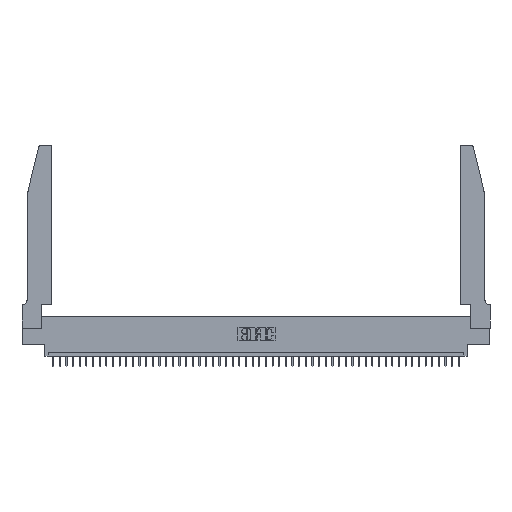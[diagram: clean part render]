
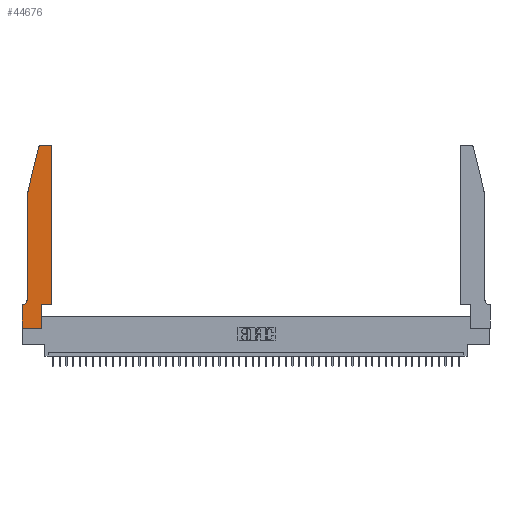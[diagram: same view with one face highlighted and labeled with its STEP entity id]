
A CAD part, top view. The second image highlights one B-rep face of the part: STEP entity #44676.
In plain terms, the highlighted planar face has unit normal (0, 0, 1).
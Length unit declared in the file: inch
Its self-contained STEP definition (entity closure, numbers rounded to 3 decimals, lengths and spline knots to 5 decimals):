
#23 = LINE ( 'NONE', #32280, #37857 ) ;
#699 = EDGE_CURVE ( 'NONE', #25619, #17878, #11691, .T. ) ;
#874 = ORIENTED_EDGE ( 'NONE', *, *, #14093, .T. ) ;
#895 = CARTESIAN_POINT ( 'NONE',  ( 0.25487, 2.72718, 0.37 ) ) ;
#1100 = CARTESIAN_POINT ( 'NONE',  ( 0.2865, 0.35, 0.37 ) ) ;
#2449 = VERTEX_POINT ( 'NONE', #40397 ) ;
#2462 = CARTESIAN_POINT ( 'NONE',  ( 0.4505, 0.35, 0.37 ) ) ;
#2941 = ORIENTED_EDGE ( 'NONE', *, *, #3847, .T. ) ;
#3013 = DIRECTION ( 'NONE',  ( 0., 1., 0. ) ) ;
#3695 = ORIENTED_EDGE ( 'NONE', *, *, #42398, .T. ) ;
#3847 = EDGE_CURVE ( 'NONE', #35915, #27266, #47450, .T. ) ;
#4477 = AXIS2_PLACEMENT_3D ( 'NONE', #24821, #9919, #25151 ) ;
#4875 = CARTESIAN_POINT ( 'NONE',  ( 0.0755, 0.42, 0.37 ) ) ;
#5432 = EDGE_LOOP ( 'NONE', ( #874, #41596, #39174, #23337, #21765, #13843, #41439, #3695, #14751, #2941, #32762, #30249 ) ) ;
#6868 = DIRECTION ( 'NONE',  ( -1., 0., 0. ) ) ;
#6948 = DIRECTION ( 'NONE',  ( 0., 1., 0. ) ) ;
#7345 = CARTESIAN_POINT ( 'NONE',  ( 0.4505, 0.35, 0.37 ) ) ;
#7988 = DIRECTION ( 'NONE',  ( 0., -1., 0. ) ) ;
#8310 = CARTESIAN_POINT ( 'NONE',  ( 0.284, 2.75, 0.37 ) ) ;
#8415 = VECTOR ( 'NONE', #6868, 39.37008 ) ;
#8465 = DIRECTION ( 'NONE',  ( 0., 0., 1. ) ) ;
#8596 = CIRCLE ( 'NONE', #4477, 0.03 ) ;
#8903 = EDGE_CURVE ( 'NONE', #35233, #26789, #16648, .T. ) ;
#9687 = VERTEX_POINT ( 'NONE', #895 ) ;
#9919 = DIRECTION ( 'NONE',  ( 0., 0., 1. ) ) ;
#10897 = LINE ( 'NONE', #25652, #37524 ) ;
#11164 = DIRECTION ( 'NONE',  ( -0.239, -0.971, 0. ) ) ;
#11323 = CARTESIAN_POINT ( 'NONE',  ( 0.0755, 2., 0.37 ) ) ;
#11691 = LINE ( 'NONE', #21975, #24125 ) ;
#12557 = DIRECTION ( 'NONE',  ( -1., 0., 0. ) ) ;
#13031 = VECTOR ( 'NONE', #11164, 39.37008 ) ;
#13135 = DIRECTION ( 'NONE',  ( 0., 0., -1. ) ) ;
#13655 = VERTEX_POINT ( 'NONE', #8310 ) ;
#13843 = ORIENTED_EDGE ( 'NONE', *, *, #21117, .T. ) ;
#14093 = EDGE_CURVE ( 'NONE', #30449, #13655, #48654, .T. ) ;
#14190 = VECTOR ( 'NONE', #26966, 39.37008 ) ;
#14314 = DIRECTION ( 'NONE',  ( 0., 0., 1. ) ) ;
#14751 = ORIENTED_EDGE ( 'NONE', *, *, #24296, .T. ) ;
#14823 = DIRECTION ( 'NONE',  ( -1., 0., 0. ) ) ;
#15380 = CARTESIAN_POINT ( 'NONE',  ( 0.4505, 0.35, 0.37 ) ) ;
#15409 = VECTOR ( 'NONE', #3013, 39.37008 ) ;
#16256 = EDGE_CURVE ( 'NONE', #13655, #9687, #17900, .T. ) ;
#16648 = LINE ( 'NONE', #24635, #34934 ) ;
#17878 = VERTEX_POINT ( 'NONE', #4875 ) ;
#17900 = CIRCLE ( 'NONE', #21139, 0.03 ) ;
#17932 = VECTOR ( 'NONE', #18370, 39.37008 ) ;
#18126 = CARTESIAN_POINT ( 'NONE',  ( 0.2605, 2.75, 0.37 ) ) ;
#18370 = DIRECTION ( 'NONE',  ( 1., 0., 0. ) ) ;
#21102 = VERTEX_POINT ( 'NONE', #45766 ) ;
#21117 = EDGE_CURVE ( 'NONE', #35911, #35233, #23, .T. ) ;
#21139 = AXIS2_PLACEMENT_3D ( 'NONE', #23509, #8465, #34865 ) ;
#21765 = ORIENTED_EDGE ( 'NONE', *, *, #27691, .T. ) ;
#21975 = CARTESIAN_POINT ( 'NONE',  ( 0.0755, 2., 0.37 ) ) ;
#22614 = CIRCLE ( 'NONE', #40969, 0.07 ) ;
#23056 = LINE ( 'NONE', #11323, #13031 ) ;
#23190 = CARTESIAN_POINT ( 'NONE',  ( 0., 0., 0.37 ) ) ;
#23337 = ORIENTED_EDGE ( 'NONE', *, *, #699, .T. ) ;
#23509 = CARTESIAN_POINT ( 'NONE',  ( 0.284, 2.72, 0.37 ) ) ;
#24125 = VECTOR ( 'NONE', #7988, 39.37008 ) ;
#24296 = EDGE_CURVE ( 'NONE', #2449, #35915, #10897, .T. ) ;
#24635 = CARTESIAN_POINT ( 'NONE',  ( 0., 0., 0.37 ) ) ;
#24821 = CARTESIAN_POINT ( 'NONE',  ( 0.4205, 2.72, 0.37 ) ) ;
#25151 = DIRECTION ( 'NONE',  ( 1., 0., 0. ) ) ;
#25487 = LINE ( 'NONE', #7345, #15409 ) ;
#25619 = VERTEX_POINT ( 'NONE', #39149 ) ;
#25652 = CARTESIAN_POINT ( 'NONE',  ( 0.2865, 0.35, 0.37 ) ) ;
#26789 = VERTEX_POINT ( 'NONE', #44577 ) ;
#26958 = AXIS2_PLACEMENT_3D ( 'NONE', #40767, #14314, #44571 ) ;
#26966 = DIRECTION ( 'NONE',  ( 1., 0., 0. ) ) ;
#27266 = VERTEX_POINT ( 'NONE', #2462 ) ;
#27691 = EDGE_CURVE ( 'NONE', #17878, #35911, #22614, .T. ) ;
#29568 = LINE ( 'NONE', #23190, #14190 ) ;
#30249 = ORIENTED_EDGE ( 'NONE', *, *, #39207, .T. ) ;
#30449 = VERTEX_POINT ( 'NONE', #38859 ) ;
#30717 = FACE_OUTER_BOUND ( 'NONE', #5432, .T. ) ;
#31787 = CARTESIAN_POINT ( 'NONE',  ( 0.0055, 0.42, 0.37 ) ) ;
#32280 = CARTESIAN_POINT ( 'NONE',  ( 0.0755, 0.35, 0.37 ) ) ;
#32762 = ORIENTED_EDGE ( 'NONE', *, *, #42264, .T. ) ;
#34865 = DIRECTION ( 'NONE',  ( 1., 0., 0. ) ) ;
#34934 = VECTOR ( 'NONE', #41010, 39.37008 ) ;
#35233 = VERTEX_POINT ( 'NONE', #47978 ) ;
#35841 = CARTESIAN_POINT ( 'NONE',  ( 0.0055, 0.35, 0.37 ) ) ;
#35911 = VERTEX_POINT ( 'NONE', #35841 ) ;
#35915 = VERTEX_POINT ( 'NONE', #1100 ) ;
#37524 = VECTOR ( 'NONE', #6948, 39.37008 ) ;
#37857 = VECTOR ( 'NONE', #12557, 39.37008 ) ;
#38859 = CARTESIAN_POINT ( 'NONE',  ( 0.4205, 2.75, 0.37 ) ) ;
#39149 = CARTESIAN_POINT ( 'NONE',  ( 0.0755, 2., 0.37 ) ) ;
#39174 = ORIENTED_EDGE ( 'NONE', *, *, #44703, .T. ) ;
#39207 = EDGE_CURVE ( 'NONE', #21102, #30449, #8596, .T. ) ;
#40397 = CARTESIAN_POINT ( 'NONE',  ( 0.2865, 0., 0.37 ) ) ;
#40767 = CARTESIAN_POINT ( 'NONE',  ( 0., 0.35, 0.37 ) ) ;
#40944 = PLANE ( 'NONE',  #26958 ) ;
#40969 = AXIS2_PLACEMENT_3D ( 'NONE', #31787, #13135, #14823 ) ;
#41010 = DIRECTION ( 'NONE',  ( 0., -1., 0. ) ) ;
#41439 = ORIENTED_EDGE ( 'NONE', *, *, #8903, .T. ) ;
#41596 = ORIENTED_EDGE ( 'NONE', *, *, #16256, .T. ) ;
#42264 = EDGE_CURVE ( 'NONE', #27266, #21102, #25487, .T. ) ;
#42398 = EDGE_CURVE ( 'NONE', #26789, #2449, #29568, .T. ) ;
#44571 = DIRECTION ( 'NONE',  ( 1., 0., 0. ) ) ;
#44577 = CARTESIAN_POINT ( 'NONE',  ( 0., 0., 0.37 ) ) ;
#44676 = ADVANCED_FACE ( 'NONE', ( #30717 ), #40944, .T. ) ;
#44703 = EDGE_CURVE ( 'NONE', #9687, #25619, #23056, .T. ) ;
#45766 = CARTESIAN_POINT ( 'NONE',  ( 0.4505, 2.72, 0.37 ) ) ;
#47450 = LINE ( 'NONE', #15380, #17932 ) ;
#47978 = CARTESIAN_POINT ( 'NONE',  ( 0., 0.35, 0.37 ) ) ;
#48654 = LINE ( 'NONE', #18126, #8415 ) ;
